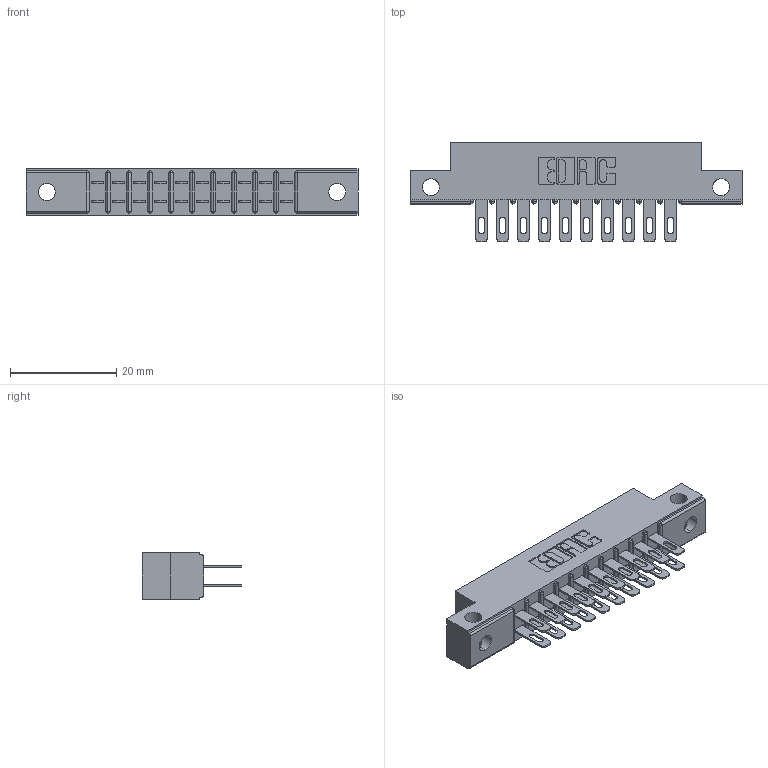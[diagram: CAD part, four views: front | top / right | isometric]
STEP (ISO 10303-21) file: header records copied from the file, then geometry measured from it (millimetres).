
FILE_DESCRIPTION (( 'STEP AP203' ), '1' );
FILE_NAME ('355-020-500-212.STEP', '2020-09-20T05:10:35', ( '' ), ( '' ), 'SwSTEP 2.0', 'SolidWorks 2020', '' );
FILE_SCHEMA (( 'CONFIG_CONTROL_DESIGN' ));
Length unit declared in the file: inch
Products named in the file (3): 305 Part_.128 Dia; 355-020-500-212; 305-290-001_500
Assembly tree (21 placements, depth 2):
  355-020-500-212
    305 Part_.128 Dia
    305-290-001_500  x20
Bounding box: 62.64 x 18.85 x 8.71 mm (x, y, z)
Volume: 3868.9 mm3; surface area: 6959.4 mm2
Topology: 21 solids, 21 shells, 1128 faces, 3222 edges, 2088 vertices
Faces by surface type: plane 628, cylinder 460, sphere 40
Entity records: 15151 total; most frequent: CARTESIAN_POINT 2556, ORIENTED_EDGE 2488, DIRECTION 2440, EDGE_CURVE 1244, LINE 952, VECTOR 952, VERTEX_POINT 796, AXIS2_PLACEMENT_3D 744
